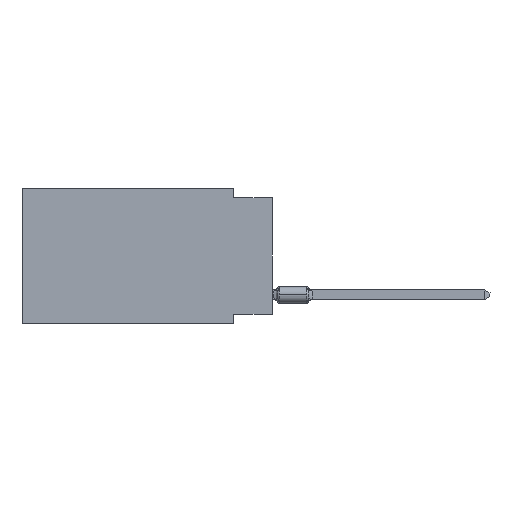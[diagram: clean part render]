
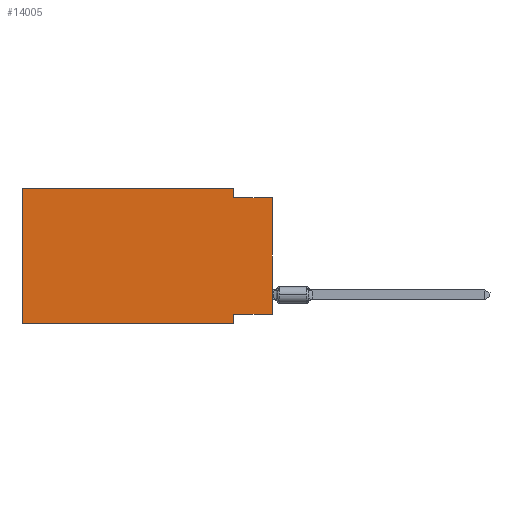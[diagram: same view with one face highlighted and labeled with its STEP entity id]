
A CAD part, left-side view. The second image highlights one B-rep face of the part: STEP entity #14005.
In plain terms, the highlighted planar face has unit normal (-1, 0, 0).
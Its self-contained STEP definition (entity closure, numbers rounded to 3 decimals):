
#213 = VECTOR ( 'NONE', #17321, 1000. ) ;
#258 = ORIENTED_EDGE ( 'NONE', *, *, #9237, .T. ) ;
#619 = DIRECTION ( 'NONE',  ( 1., 0., 0. ) ) ;
#1218 = EDGE_CURVE ( 'NONE', #10448, #2435, #3601, .T. ) ;
#1249 = DIRECTION ( 'NONE',  ( 0., 1., 0. ) ) ;
#1762 = ORIENTED_EDGE ( 'NONE', *, *, #10283, .F. ) ;
#2435 = VERTEX_POINT ( 'NONE', #20883 ) ;
#3072 = LINE ( 'NONE', #10873, #213 ) ;
#3480 = ORIENTED_EDGE ( 'NONE', *, *, #6472, .F. ) ;
#3601 = LINE ( 'NONE', #10355, #12956 ) ;
#3859 = CARTESIAN_POINT ( 'NONE',  ( 0., 16.383, 0. ) ) ;
#4376 = DIRECTION ( 'NONE',  ( 0., 0., -1. ) ) ;
#4428 = LINE ( 'NONE', #15722, #12366 ) ;
#4584 = VERTEX_POINT ( 'NONE', #16495 ) ;
#5162 = VECTOR ( 'NONE', #11504, 1000. ) ;
#5170 = EDGE_CURVE ( 'NONE', #4584, #2435, #10331, .T. ) ;
#5506 = ORIENTED_EDGE ( 'NONE', *, *, #10752, .F. ) ;
#5770 = CARTESIAN_POINT ( 'NONE',  ( 0., 16.383, 0. ) ) ;
#6034 = DIRECTION ( 'NONE',  ( 0., -1., 0. ) ) ;
#6162 = CARTESIAN_POINT ( 'NONE',  ( 0., 2.54, -8.89 ) ) ;
#6472 = EDGE_CURVE ( 'NONE', #14985, #12476, #19148, .T. ) ;
#8550 = CARTESIAN_POINT ( 'NONE',  ( 0., 16.383, 0. ) ) ;
#8640 = VERTEX_POINT ( 'NONE', #10319 ) ;
#8688 = DIRECTION ( 'NONE',  ( 0., -1., 0. ) ) ;
#9215 = CARTESIAN_POINT ( 'NONE',  ( 0., 2.54, -8.255 ) ) ;
#9237 = EDGE_CURVE ( 'NONE', #13763, #12476, #11398, .T. ) ;
#9817 = CARTESIAN_POINT ( 'NONE',  ( 0., 2.54, -0.635 ) ) ;
#9902 = DIRECTION ( 'NONE',  ( 0., 0., -1. ) ) ;
#9906 = CARTESIAN_POINT ( 'NONE',  ( 0., 16.383, -8.89 ) ) ;
#10283 = EDGE_CURVE ( 'NONE', #8640, #10448, #3072, .T. ) ;
#10319 = CARTESIAN_POINT ( 'NONE',  ( 0., 2.54, 0. ) ) ;
#10331 = LINE ( 'NONE', #10437, #16862 ) ;
#10355 = CARTESIAN_POINT ( 'NONE',  ( 0., 0., -0.635 ) ) ;
#10437 = CARTESIAN_POINT ( 'NONE',  ( 0., 0., 0. ) ) ;
#10448 = VERTEX_POINT ( 'NONE', #9817 ) ;
#10752 = EDGE_CURVE ( 'NONE', #4584, #14985, #4428, .T. ) ;
#10873 = CARTESIAN_POINT ( 'NONE',  ( 0., 2.54, 0. ) ) ;
#11398 = LINE ( 'NONE', #9906, #5162 ) ;
#11504 = DIRECTION ( 'NONE',  ( 0., -1., 0. ) ) ;
#12366 = VECTOR ( 'NONE', #1249, 1000. ) ;
#12476 = VERTEX_POINT ( 'NONE', #13471 ) ;
#12606 = AXIS2_PLACEMENT_3D ( 'NONE', #8550, #619, #9902 ) ;
#12956 = VECTOR ( 'NONE', #8688, 1000. ) ;
#13288 = FACE_OUTER_BOUND ( 'NONE', #15460, .T. ) ;
#13471 = CARTESIAN_POINT ( 'NONE',  ( 0., 2.54, -8.89 ) ) ;
#13742 = EDGE_CURVE ( 'NONE', #19783, #8640, #20611, .T. ) ;
#13763 = VERTEX_POINT ( 'NONE', #17017 ) ;
#13859 = VECTOR ( 'NONE', #16755, 1000. ) ;
#14005 = ADVANCED_FACE ( 'NONE', ( #13288 ), #20059, .F. ) ;
#14985 = VERTEX_POINT ( 'NONE', #9215 ) ;
#15460 = EDGE_LOOP ( 'NONE', ( #18093, #20433, #1762, #16906, #15872, #258, #3480, #5506 ) ) ;
#15721 = VECTOR ( 'NONE', #4376, 1000. ) ;
#15722 = CARTESIAN_POINT ( 'NONE',  ( 0., 0., -8.255 ) ) ;
#15872 = ORIENTED_EDGE ( 'NONE', *, *, #19705, .F. ) ;
#16495 = CARTESIAN_POINT ( 'NONE',  ( 0., 0., -8.255 ) ) ;
#16755 = DIRECTION ( 'NONE',  ( 0., 0., 1. ) ) ;
#16784 = DIRECTION ( 'NONE',  ( 0., 0., 1. ) ) ;
#16862 = VECTOR ( 'NONE', #16784, 1000. ) ;
#16906 = ORIENTED_EDGE ( 'NONE', *, *, #13742, .F. ) ;
#17017 = CARTESIAN_POINT ( 'NONE',  ( 0., 16.383, -8.89 ) ) ;
#17123 = CARTESIAN_POINT ( 'NONE',  ( 0., 16.383, 0. ) ) ;
#17321 = DIRECTION ( 'NONE',  ( 0., 0., -1. ) ) ;
#18093 = ORIENTED_EDGE ( 'NONE', *, *, #5170, .T. ) ;
#18328 = LINE ( 'NONE', #3859, #13859 ) ;
#19148 = LINE ( 'NONE', #6162, #15721 ) ;
#19376 = VECTOR ( 'NONE', #6034, 1000. ) ;
#19705 = EDGE_CURVE ( 'NONE', #13763, #19783, #18328, .T. ) ;
#19783 = VERTEX_POINT ( 'NONE', #5770 ) ;
#20059 = PLANE ( 'NONE',  #12606 ) ;
#20433 = ORIENTED_EDGE ( 'NONE', *, *, #1218, .F. ) ;
#20611 = LINE ( 'NONE', #17123, #19376 ) ;
#20883 = CARTESIAN_POINT ( 'NONE',  ( 0., 0., -0.635 ) ) ;
